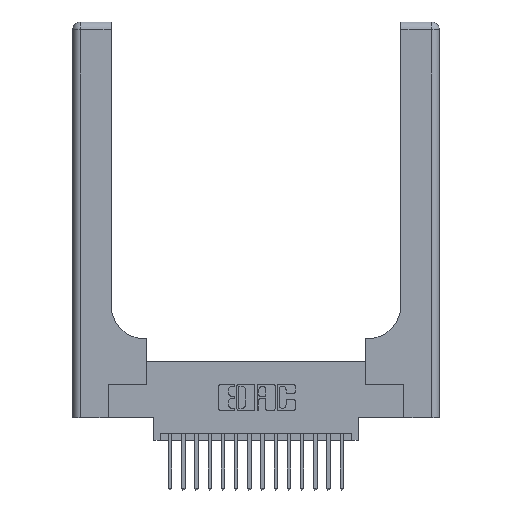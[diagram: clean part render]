
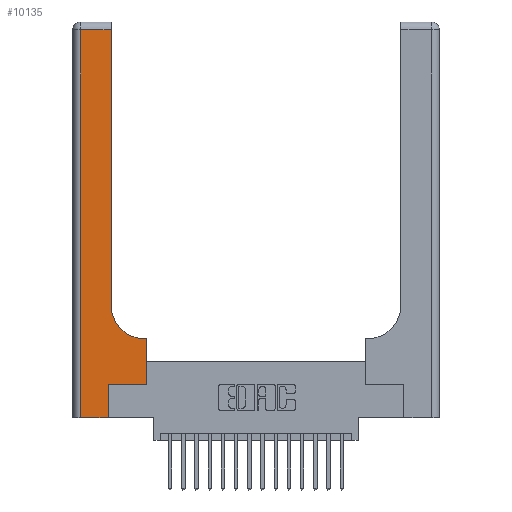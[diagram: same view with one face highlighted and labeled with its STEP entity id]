
A CAD part, top view. The second image highlights one B-rep face of the part: STEP entity #10135.
In plain terms, the highlighted planar face has unit normal (0, 0, 1).
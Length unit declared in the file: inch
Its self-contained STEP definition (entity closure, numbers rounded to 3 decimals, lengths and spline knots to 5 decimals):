
#360 = LINE ( 'NONE', #6096, #2041 ) ;
#599 = ORIENTED_EDGE ( 'NONE', *, *, #6613, .T. ) ;
#1050 = VERTEX_POINT ( 'NONE', #13709 ) ;
#1606 = CARTESIAN_POINT ( 'NONE',  ( 0.2915, 3., 0.37 ) ) ;
#1690 = EDGE_CURVE ( 'NONE', #18529, #1050, #4609, .T. ) ;
#1757 = CARTESIAN_POINT ( 'NONE',  ( 0.269, 0., 0.37 ) ) ;
#1774 = ORIENTED_EDGE ( 'NONE', *, *, #2317, .T. ) ;
#2041 = VECTOR ( 'NONE', #10485, 39.37008 ) ;
#2310 = LINE ( 'NONE', #9393, #13952 ) ;
#2317 = EDGE_CURVE ( 'NONE', #16292, #16840, #15778, .T. ) ;
#2855 = VECTOR ( 'NONE', #15483, 39.37008 ) ;
#2892 = VECTOR ( 'NONE', #12464, 39.37008 ) ;
#3182 = EDGE_CURVE ( 'NONE', #15591, #14111, #8241, .T. ) ;
#3622 = EDGE_CURVE ( 'NONE', #1050, #5871, #7019, .T. ) ;
#3724 = DIRECTION ( 'NONE',  ( 0., 1., 0. ) ) ;
#3847 = CARTESIAN_POINT ( 'NONE',  ( 0.06, 2.94, 0.37 ) ) ;
#4501 = PLANE ( 'NONE',  #9337 ) ;
#4609 = LINE ( 'NONE', #12981, #9755 ) ;
#4729 = CARTESIAN_POINT ( 'NONE',  ( 0.2915, 0.85, 0.37 ) ) ;
#4879 = DIRECTION ( 'NONE',  ( 1., 0., 0. ) ) ;
#4902 = CIRCLE ( 'NONE', #7120, 0.25 ) ;
#5349 = VERTEX_POINT ( 'NONE', #3847 ) ;
#5871 = VERTEX_POINT ( 'NONE', #13904 ) ;
#6096 = CARTESIAN_POINT ( 'NONE',  ( 0., 2.94, 0.37 ) ) ;
#6613 = EDGE_CURVE ( 'NONE', #5349, #16292, #10782, .T. ) ;
#6670 = VECTOR ( 'NONE', #16557, 39.37008 ) ;
#7019 = LINE ( 'NONE', #12286, #2855 ) ;
#7120 = AXIS2_PLACEMENT_3D ( 'NONE', #11026, #14213, #17299 ) ;
#8241 = LINE ( 'NONE', #1606, #2892 ) ;
#8849 = ORIENTED_EDGE ( 'NONE', *, *, #3622, .T. ) ;
#8964 = DIRECTION ( 'NONE',  ( 0., 0., -1. ) ) ;
#9337 = AXIS2_PLACEMENT_3D ( 'NONE', #11984, #8964, #19815 ) ;
#9393 = CARTESIAN_POINT ( 'NONE',  ( 0.269, 0.25, 0.37 ) ) ;
#9399 = VECTOR ( 'NONE', #13471, 39.37008 ) ;
#9755 = VECTOR ( 'NONE', #3724, 39.37008 ) ;
#9827 = EDGE_CURVE ( 'NONE', #16792, #18529, #2310, .T. ) ;
#10135 = ADVANCED_FACE ( 'NONE', ( #20070 ), #4501, .F. ) ;
#10404 = DIRECTION ( 'NONE',  ( 1., 0., 0. ) ) ;
#10485 = DIRECTION ( 'NONE',  ( -1., 0., 0. ) ) ;
#10782 = LINE ( 'NONE', #15195, #6670 ) ;
#10796 = EDGE_LOOP ( 'NONE', ( #17789, #15909, #599, #1774, #14599, #15222, #11372, #8849, #14764 ) ) ;
#11026 = CARTESIAN_POINT ( 'NONE',  ( 0.5415, 0.85, 0.37 ) ) ;
#11372 = ORIENTED_EDGE ( 'NONE', *, *, #1690, .T. ) ;
#11984 = CARTESIAN_POINT ( 'NONE',  ( 0., 3., 0.37 ) ) ;
#12274 = CARTESIAN_POINT ( 'NONE',  ( 0.5585, 0.25, 0.37 ) ) ;
#12286 = CARTESIAN_POINT ( 'NONE',  ( 0.2915, 0.6, 0.37 ) ) ;
#12464 = DIRECTION ( 'NONE',  ( 0., 1., 0. ) ) ;
#12684 = CARTESIAN_POINT ( 'NONE',  ( 0.269, 0.25, 0.37 ) ) ;
#12981 = CARTESIAN_POINT ( 'NONE',  ( 0.5585, 0.25, 0.37 ) ) ;
#13471 = DIRECTION ( 'NONE',  ( 0., 1., 0. ) ) ;
#13535 = CARTESIAN_POINT ( 'NONE',  ( 0.269, 0., 0.37 ) ) ;
#13709 = CARTESIAN_POINT ( 'NONE',  ( 0.5585, 0.6, 0.37 ) ) ;
#13904 = CARTESIAN_POINT ( 'NONE',  ( 0.5415, 0.6, 0.37 ) ) ;
#13952 = VECTOR ( 'NONE', #4879, 39.37008 ) ;
#13988 = LINE ( 'NONE', #13535, #9399 ) ;
#14111 = VERTEX_POINT ( 'NONE', #18059 ) ;
#14213 = DIRECTION ( 'NONE',  ( 0., 0., -1. ) ) ;
#14599 = ORIENTED_EDGE ( 'NONE', *, *, #16478, .T. ) ;
#14764 = ORIENTED_EDGE ( 'NONE', *, *, #19629, .T. ) ;
#15195 = CARTESIAN_POINT ( 'NONE',  ( 0.06, 3., 0.37 ) ) ;
#15222 = ORIENTED_EDGE ( 'NONE', *, *, #9827, .T. ) ;
#15483 = DIRECTION ( 'NONE',  ( -1., 0., 0. ) ) ;
#15534 = VECTOR ( 'NONE', #10404, 39.37008 ) ;
#15591 = VERTEX_POINT ( 'NONE', #4729 ) ;
#15778 = LINE ( 'NONE', #16473, #15534 ) ;
#15909 = ORIENTED_EDGE ( 'NONE', *, *, #18950, .T. ) ;
#16292 = VERTEX_POINT ( 'NONE', #19021 ) ;
#16473 = CARTESIAN_POINT ( 'NONE',  ( 0., 0., 0.37 ) ) ;
#16478 = EDGE_CURVE ( 'NONE', #16840, #16792, #13988, .T. ) ;
#16557 = DIRECTION ( 'NONE',  ( 0., -1., 0. ) ) ;
#16792 = VERTEX_POINT ( 'NONE', #12684 ) ;
#16840 = VERTEX_POINT ( 'NONE', #1757 ) ;
#17299 = DIRECTION ( 'NONE',  ( 1., 0., 0. ) ) ;
#17789 = ORIENTED_EDGE ( 'NONE', *, *, #3182, .T. ) ;
#18059 = CARTESIAN_POINT ( 'NONE',  ( 0.2915, 2.94, 0.37 ) ) ;
#18529 = VERTEX_POINT ( 'NONE', #12274 ) ;
#18950 = EDGE_CURVE ( 'NONE', #14111, #5349, #360, .T. ) ;
#19021 = CARTESIAN_POINT ( 'NONE',  ( 0.06, 0., 0.37 ) ) ;
#19629 = EDGE_CURVE ( 'NONE', #5871, #15591, #4902, .T. ) ;
#19815 = DIRECTION ( 'NONE',  ( -1., 0., 0. ) ) ;
#20070 = FACE_OUTER_BOUND ( 'NONE', #10796, .T. ) ;
